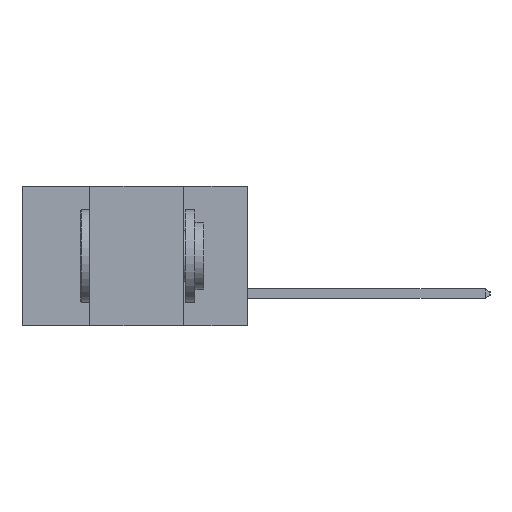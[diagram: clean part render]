
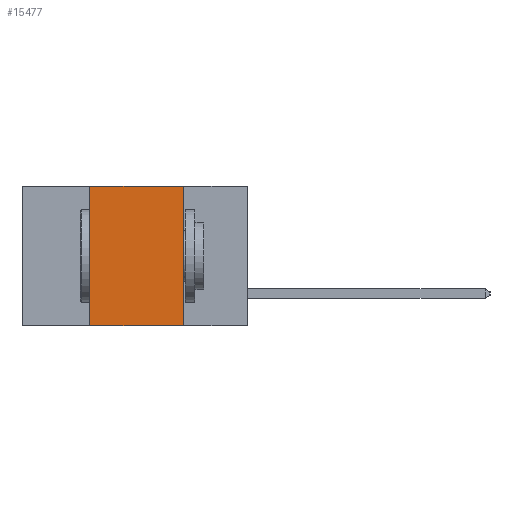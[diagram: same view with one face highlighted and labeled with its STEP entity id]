
A CAD part, left-side view. The second image highlights one B-rep face of the part: STEP entity #15477.
In plain terms, the highlighted planar face has unit normal (-1, 0, 0).
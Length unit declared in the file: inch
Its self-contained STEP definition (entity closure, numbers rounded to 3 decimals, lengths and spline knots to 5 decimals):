
#166 = EDGE_LOOP ( 'NONE', ( #17990, #23212, #20654, #24078 ) ) ;
#216 = DIRECTION ( 'NONE',  ( 0., -1., 0. ) ) ;
#302 = CARTESIAN_POINT ( 'NONE',  ( 0., 0.6, 0. ) ) ;
#1067 = CARTESIAN_POINT ( 'NONE',  ( 0., 0.42, -0.37 ) ) ;
#1137 = EDGE_CURVE ( 'NONE', #24531, #3771, #23708, .T. ) ;
#1754 = CARTESIAN_POINT ( 'NONE',  ( 0., 0.42, -0.37 ) ) ;
#1994 = EDGE_CURVE ( 'NONE', #3090, #9462, #13132, .T. ) ;
#3090 = VERTEX_POINT ( 'NONE', #1067 ) ;
#3664 = DIRECTION ( 'NONE',  ( 1., 0., 0. ) ) ;
#3771 = VERTEX_POINT ( 'NONE', #20423 ) ;
#4728 = VECTOR ( 'NONE', #16004, 39.37008 ) ;
#5572 = CARTESIAN_POINT ( 'NONE',  ( 0., 0.17, 0. ) ) ;
#8980 = LINE ( 'NONE', #302, #13583 ) ;
#9462 = VERTEX_POINT ( 'NONE', #18795 ) ;
#13132 = LINE ( 'NONE', #1754, #17600 ) ;
#13193 = EDGE_CURVE ( 'NONE', #9462, #24531, #8980, .T. ) ;
#13583 = VECTOR ( 'NONE', #216, 39.37008 ) ;
#14073 = DIRECTION ( 'NONE',  ( 0., 0., 1. ) ) ;
#14074 = CARTESIAN_POINT ( 'NONE',  ( 0., 0.6, -0.37 ) ) ;
#14547 = CARTESIAN_POINT ( 'NONE',  ( 0., 0.17, -0.37 ) ) ;
#15477 = ADVANCED_FACE ( 'NONE', ( #24794 ), #24689, .F. ) ;
#16004 = DIRECTION ( 'NONE',  ( 0., -1., 0. ) ) ;
#17040 = VECTOR ( 'NONE', #18389, 39.37008 ) ;
#17390 = DIRECTION ( 'NONE',  ( 0., 0., -1. ) ) ;
#17600 = VECTOR ( 'NONE', #14073, 39.37008 ) ;
#17990 = ORIENTED_EDGE ( 'NONE', *, *, #1137, .F. ) ;
#18389 = DIRECTION ( 'NONE',  ( 0., 0., -1. ) ) ;
#18795 = CARTESIAN_POINT ( 'NONE',  ( 0., 0.42, 0. ) ) ;
#19202 = CARTESIAN_POINT ( 'NONE',  ( 0., 0.6, 0. ) ) ;
#19539 = AXIS2_PLACEMENT_3D ( 'NONE', #19202, #3664, #17390 ) ;
#20235 = LINE ( 'NONE', #14074, #4728 ) ;
#20423 = CARTESIAN_POINT ( 'NONE',  ( 0., 0.17, -0.37 ) ) ;
#20654 = ORIENTED_EDGE ( 'NONE', *, *, #1994, .F. ) ;
#22940 = EDGE_CURVE ( 'NONE', #3090, #3771, #20235, .T. ) ;
#23212 = ORIENTED_EDGE ( 'NONE', *, *, #13193, .F. ) ;
#23708 = LINE ( 'NONE', #14547, #17040 ) ;
#24078 = ORIENTED_EDGE ( 'NONE', *, *, #22940, .T. ) ;
#24531 = VERTEX_POINT ( 'NONE', #5572 ) ;
#24689 = PLANE ( 'NONE',  #19539 ) ;
#24794 = FACE_OUTER_BOUND ( 'NONE', #166, .T. ) ;
